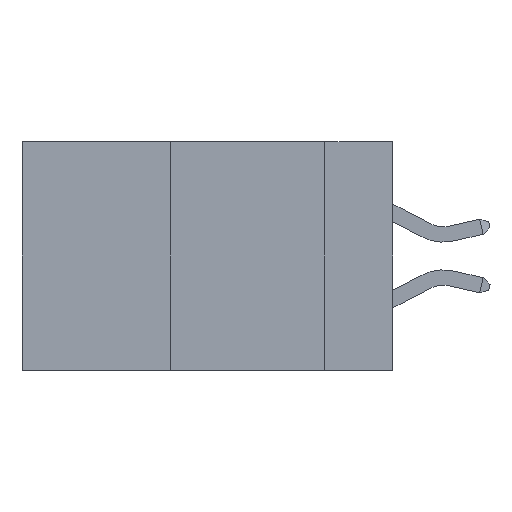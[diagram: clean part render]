
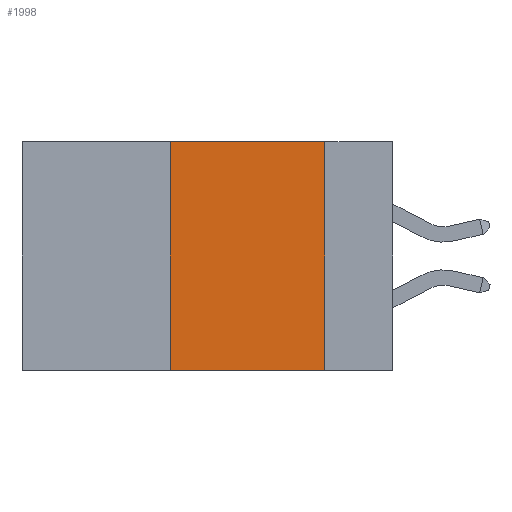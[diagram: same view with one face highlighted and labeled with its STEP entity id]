
A CAD part, left-side view. The second image highlights one B-rep face of the part: STEP entity #1998.
In plain terms, the highlighted planar face has unit normal (-1, 0, 0).
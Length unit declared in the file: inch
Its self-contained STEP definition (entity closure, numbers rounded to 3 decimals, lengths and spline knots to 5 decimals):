
#881 = EDGE_CURVE ( 'NONE', #4757, #14158, #11036, .T. ) ;
#1011 = CARTESIAN_POINT ( 'NONE',  ( 0., 0.36, 0. ) ) ;
#1258 = VECTOR ( 'NONE', #13971, 39.37008 ) ;
#1288 = CARTESIAN_POINT ( 'NONE',  ( 0., 0.11, 0. ) ) ;
#1368 = DIRECTION ( 'NONE',  ( 0., 0., -1. ) ) ;
#1750 = EDGE_CURVE ( 'NONE', #7248, #4255, #2695, .T. ) ;
#1998 = ADVANCED_FACE ( 'NONE', ( #14652 ), #3604, .F. ) ;
#2695 = LINE ( 'NONE', #1288, #1258 ) ;
#2879 = EDGE_CURVE ( 'NONE', #4757, #4255, #13526, .T. ) ;
#3303 = DIRECTION ( 'NONE',  ( 0., 0., 1. ) ) ;
#3604 = PLANE ( 'NONE',  #13147 ) ;
#3940 = CARTESIAN_POINT ( 'NONE',  ( 0., 0.36, -0.37 ) ) ;
#4255 = VERTEX_POINT ( 'NONE', #11831 ) ;
#4605 = CARTESIAN_POINT ( 'NONE',  ( 0., 0.6, 0. ) ) ;
#4757 = VERTEX_POINT ( 'NONE', #3940 ) ;
#6125 = VECTOR ( 'NONE', #7972, 39.37008 ) ;
#6269 = VECTOR ( 'NONE', #7934, 39.37008 ) ;
#6439 = CARTESIAN_POINT ( 'NONE',  ( 0., 0.36, 0. ) ) ;
#6510 = ORIENTED_EDGE ( 'NONE', *, *, #1750, .F. ) ;
#7248 = VERTEX_POINT ( 'NONE', #7273 ) ;
#7273 = CARTESIAN_POINT ( 'NONE',  ( 0., 0.11, 0. ) ) ;
#7793 = EDGE_LOOP ( 'NONE', ( #6510, #9331, #10308, #11459 ) ) ;
#7934 = DIRECTION ( 'NONE',  ( 0., -1., 0. ) ) ;
#7972 = DIRECTION ( 'NONE',  ( 0., -1., 0. ) ) ;
#8137 = CARTESIAN_POINT ( 'NONE',  ( 0., 0.6, -0.37 ) ) ;
#9005 = LINE ( 'NONE', #4605, #6125 ) ;
#9331 = ORIENTED_EDGE ( 'NONE', *, *, #11756, .F. ) ;
#10308 = ORIENTED_EDGE ( 'NONE', *, *, #881, .F. ) ;
#11036 = LINE ( 'NONE', #1011, #12125 ) ;
#11459 = ORIENTED_EDGE ( 'NONE', *, *, #2879, .T. ) ;
#11756 = EDGE_CURVE ( 'NONE', #14158, #7248, #9005, .T. ) ;
#11831 = CARTESIAN_POINT ( 'NONE',  ( 0., 0.11, -0.37 ) ) ;
#12125 = VECTOR ( 'NONE', #3303, 39.37008 ) ;
#12869 = CARTESIAN_POINT ( 'NONE',  ( 0., 0.6, 0. ) ) ;
#12922 = DIRECTION ( 'NONE',  ( 1., 0., 0. ) ) ;
#13147 = AXIS2_PLACEMENT_3D ( 'NONE', #12869, #12922, #1368 ) ;
#13526 = LINE ( 'NONE', #8137, #6269 ) ;
#13971 = DIRECTION ( 'NONE',  ( 0., 0., -1. ) ) ;
#14158 = VERTEX_POINT ( 'NONE', #6439 ) ;
#14652 = FACE_OUTER_BOUND ( 'NONE', #7793, .T. ) ;
